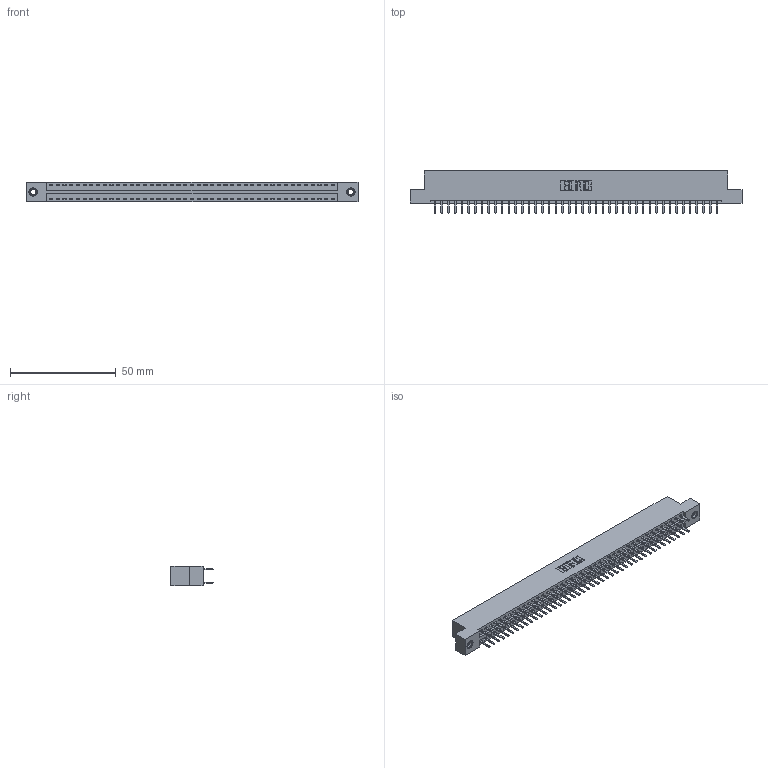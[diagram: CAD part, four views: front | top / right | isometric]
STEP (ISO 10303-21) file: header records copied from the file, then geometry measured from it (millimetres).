
FILE_DESCRIPTION (( 'STEP AP203' ), '1' );
FILE_NAME ('346-086-520-207.STEP', '2018-08-29T22:12:16', ( '' ), ( '' ), 'SwSTEP 2.0', 'SolidWorks 2016', '' );
FILE_SCHEMA (( 'CONFIG_CONTROL_DESIGN' ));
Length unit declared in the file: inch
Products named in the file (4): 346 Part_Flush Mounting Lugs - 0.156 Dia-TI; 345-292-001_345-293-120; 345-250-001_345-250-005-103; 346-086-520-207
Assembly tree (89 placements, depth 2):
  346-086-520-207
    346 Part_Flush Mounting Lugs - 0.156 Dia-TI
    345-292-001_345-293-120  x86
    345-250-001_345-250-005-103  x2
Bounding box: 157.1 x 20.02 x 9.4 mm (x, y, z)
Volume: 15275.5 mm3; surface area: 20958.2 mm2
Topology: 89 solids, 89 shells, 4998 faces, 14483 edges, 9418 vertices
Faces by surface type: plane 3290, cylinder 1692, cone 12, torus 4
Entity records: 29228 total; most frequent: CARTESIAN_POINT 4811, ORIENTED_EDGE 4726, DIRECTION 4305, EDGE_CURVE 2363, LINE 2035, VECTOR 2035, VERTEX_POINT 1568, AXIS2_PLACEMENT_3D 1135
